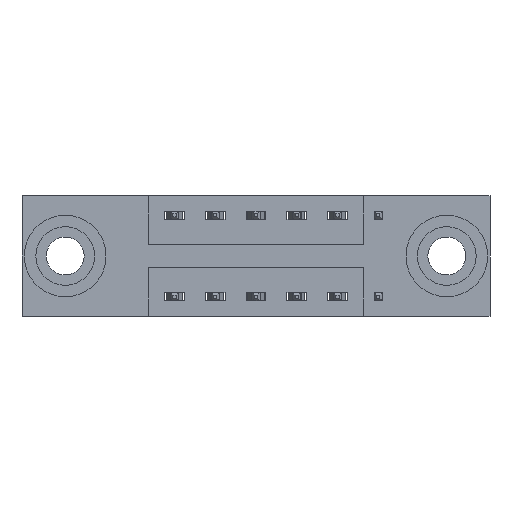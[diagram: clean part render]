
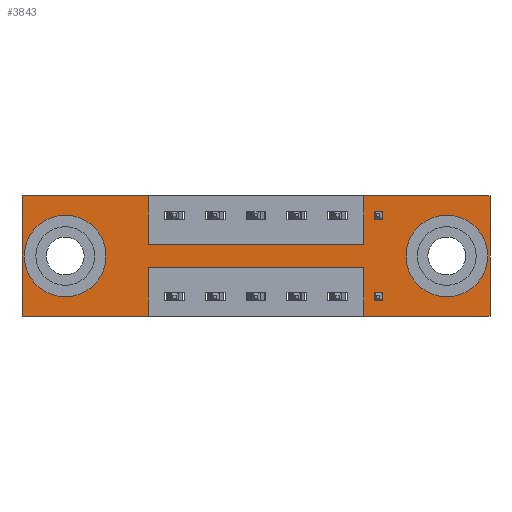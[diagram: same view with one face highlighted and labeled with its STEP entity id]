
A CAD part, front view. The second image highlights one B-rep face of the part: STEP entity #3843.
In plain terms, the highlighted planar face has unit normal (0, -1, 0).
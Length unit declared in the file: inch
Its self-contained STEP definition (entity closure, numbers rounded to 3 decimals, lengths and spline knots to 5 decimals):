
#69 = ORIENTED_EDGE ( 'NONE', *, *, #7215, .F. ) ;
#124 = DIRECTION ( 'NONE',  ( 0., 1., 0. ) ) ;
#180 = EDGE_CURVE ( 'NONE', #1295, #4848, #5429, .T. ) ;
#221 = CARTESIAN_POINT ( 'NONE',  ( 0., 0., -0.37 ) ) ;
#289 = EDGE_LOOP ( 'NONE', ( #3322, #6842, #1439, #1533, #9159, #69, #3144, #7101, #3628, #953, #3775, #3392 ) ) ;
#499 = VERTEX_POINT ( 'NONE', #5935 ) ;
#575 = DIRECTION ( 'NONE',  ( 0., 0., 1. ) ) ;
#671 = LINE ( 'NONE', #8808, #6575 ) ;
#814 = CARTESIAN_POINT ( 'NONE',  ( 0., 0., 0. ) ) ;
#820 = CARTESIAN_POINT ( 'NONE',  ( 1.0475, 0., -0.15 ) ) ;
#825 = EDGE_CURVE ( 'NONE', #3802, #5797, #4460, .T. ) ;
#881 = LINE ( 'NONE', #5229, #1136 ) ;
#882 = EDGE_CURVE ( 'NONE', #4845, #5880, #881, .T. ) ;
#922 = DIRECTION ( 'NONE',  ( 0., 0., 1. ) ) ;
#953 = ORIENTED_EDGE ( 'NONE', *, *, #7988, .F. ) ;
#956 = DIRECTION ( 'NONE',  ( -1., 0., 0. ) ) ;
#1047 = ORIENTED_EDGE ( 'NONE', *, *, #5486, .T. ) ;
#1136 = VECTOR ( 'NONE', #1576, 39.37008 ) ;
#1208 = CARTESIAN_POINT ( 'NONE',  ( 1.435, 0., -0.37 ) ) ;
#1213 = VERTEX_POINT ( 'NONE', #4296 ) ;
#1257 = EDGE_LOOP ( 'NONE', ( #1047, #8775 ) ) ;
#1295 = VERTEX_POINT ( 'NONE', #7350 ) ;
#1338 = DIRECTION ( 'NONE',  ( 0., 0., 1. ) ) ;
#1348 = DIRECTION ( 'NONE',  ( 0., 1., 0. ) ) ;
#1439 = ORIENTED_EDGE ( 'NONE', *, *, #825, .F. ) ;
#1474 = VERTEX_POINT ( 'NONE', #1208 ) ;
#1533 = ORIENTED_EDGE ( 'NONE', *, *, #3682, .F. ) ;
#1576 = DIRECTION ( 'NONE',  ( 1., 0., 0. ) ) ;
#1707 = VERTEX_POINT ( 'NONE', #9294 ) ;
#1776 = ORIENTED_EDGE ( 'NONE', *, *, #180, .T. ) ;
#1983 = EDGE_CURVE ( 'NONE', #2358, #1213, #5706, .T. ) ;
#2044 = CARTESIAN_POINT ( 'NONE',  ( 0., 0., -0.37 ) ) ;
#2072 = DIRECTION ( 'NONE',  ( 0., 0., -1. ) ) ;
#2266 = LINE ( 'NONE', #3748, #4459 ) ;
#2354 = CARTESIAN_POINT ( 'NONE',  ( 1.0475, 0., -0.37 ) ) ;
#2358 = VERTEX_POINT ( 'NONE', #4408 ) ;
#2485 = CIRCLE ( 'NONE', #9288, 0.078 ) ;
#2624 = VERTEX_POINT ( 'NONE', #6825 ) ;
#2844 = CARTESIAN_POINT ( 'NONE',  ( 0.1325, 0., -0.185 ) ) ;
#2926 = DIRECTION ( 'NONE',  ( 0., 0., -1. ) ) ;
#3001 = VECTOR ( 'NONE', #7055, 39.37008 ) ;
#3065 = DIRECTION ( 'NONE',  ( 0., 0., -1. ) ) ;
#3144 = ORIENTED_EDGE ( 'NONE', *, *, #5821, .F. ) ;
#3250 = EDGE_CURVE ( 'NONE', #7354, #1707, #6542, .T. ) ;
#3322 = ORIENTED_EDGE ( 'NONE', *, *, #3552, .F. ) ;
#3346 = FACE_OUTER_BOUND ( 'NONE', #289, .T. ) ;
#3392 = ORIENTED_EDGE ( 'NONE', *, *, #1983, .F. ) ;
#3408 = CARTESIAN_POINT ( 'NONE',  ( 0., 0., 0. ) ) ;
#3552 = EDGE_CURVE ( 'NONE', #7711, #2358, #2266, .T. ) ;
#3562 = CARTESIAN_POINT ( 'NONE',  ( 1.0475, 0., -0.22 ) ) ;
#3628 = ORIENTED_EDGE ( 'NONE', *, *, #4760, .F. ) ;
#3682 = EDGE_CURVE ( 'NONE', #1474, #3802, #3893, .T. ) ;
#3699 = EDGE_LOOP ( 'NONE', ( #8478, #1776 ) ) ;
#3748 = CARTESIAN_POINT ( 'NONE',  ( 0.3875, 0., -0.37 ) ) ;
#3775 = ORIENTED_EDGE ( 'NONE', *, *, #7913, .F. ) ;
#3802 = VERTEX_POINT ( 'NONE', #6943 ) ;
#3821 = CARTESIAN_POINT ( 'NONE',  ( 1.435, 0., 0. ) ) ;
#3843 = ADVANCED_FACE ( 'NONE', ( #8562, #9128, #3346 ), #6281, .T. ) ;
#3875 = CIRCLE ( 'NONE', #5547, 0.078 ) ;
#3893 = LINE ( 'NONE', #221, #5077 ) ;
#3953 = CARTESIAN_POINT ( 'NONE',  ( 1.3025, 0., -0.107 ) ) ;
#3959 = VECTOR ( 'NONE', #5259, 39.37008 ) ;
#4190 = DIRECTION ( 'NONE',  ( 0., 1., 0. ) ) ;
#4296 = CARTESIAN_POINT ( 'NONE',  ( 0., 0., -0.37 ) ) ;
#4347 = VECTOR ( 'NONE', #7044, 39.37008 ) ;
#4399 = CARTESIAN_POINT ( 'NONE',  ( 1.3025, 0., -0.185 ) ) ;
#4408 = CARTESIAN_POINT ( 'NONE',  ( 0.3875, 0., -0.37 ) ) ;
#4459 = VECTOR ( 'NONE', #2926, 39.37008 ) ;
#4460 = LINE ( 'NONE', #2354, #5435 ) ;
#4559 = CARTESIAN_POINT ( 'NONE',  ( 1.3025, 0., -0.185 ) ) ;
#4616 = LINE ( 'NONE', #7475, #6516 ) ;
#4716 = CARTESIAN_POINT ( 'NONE',  ( 0.3875, 0., -0.15 ) ) ;
#4757 = AXIS2_PLACEMENT_3D ( 'NONE', #2844, #4190, #1338 ) ;
#4760 = EDGE_CURVE ( 'NONE', #6452, #4845, #671, .T. ) ;
#4767 = LINE ( 'NONE', #7628, #9231 ) ;
#4845 = VERTEX_POINT ( 'NONE', #4716 ) ;
#4848 = VERTEX_POINT ( 'NONE', #3953 ) ;
#5061 = DIRECTION ( 'NONE',  ( 0., 0., -1. ) ) ;
#5065 = EDGE_CURVE ( 'NONE', #4848, #1295, #2485, .T. ) ;
#5077 = VECTOR ( 'NONE', #7505, 39.37008 ) ;
#5100 = DIRECTION ( 'NONE',  ( 0., 0., -1. ) ) ;
#5218 = CARTESIAN_POINT ( 'NONE',  ( 1.0475, 0., 0. ) ) ;
#5229 = CARTESIAN_POINT ( 'NONE',  ( 0.3875, 0., -0.15 ) ) ;
#5258 = VECTOR ( 'NONE', #922, 39.37008 ) ;
#5259 = DIRECTION ( 'NONE',  ( 0., 0., 1. ) ) ;
#5343 = LINE ( 'NONE', #814, #3959 ) ;
#5429 = CIRCLE ( 'NONE', #7054, 0.078 ) ;
#5435 = VECTOR ( 'NONE', #8832, 39.37008 ) ;
#5486 = EDGE_CURVE ( 'NONE', #1707, #7354, #3875, .T. ) ;
#5547 = AXIS2_PLACEMENT_3D ( 'NONE', #5757, #1348, #575 ) ;
#5687 = DIRECTION ( 'NONE',  ( 0., -1., 0. ) ) ;
#5706 = LINE ( 'NONE', #2044, #3001 ) ;
#5757 = CARTESIAN_POINT ( 'NONE',  ( 0.1325, 0., -0.185 ) ) ;
#5797 = VERTEX_POINT ( 'NONE', #3562 ) ;
#5821 = EDGE_CURVE ( 'NONE', #5880, #499, #8816, .T. ) ;
#5880 = VERTEX_POINT ( 'NONE', #820 ) ;
#5935 = CARTESIAN_POINT ( 'NONE',  ( 1.0475, 0., 0. ) ) ;
#6129 = EDGE_CURVE ( 'NONE', #2624, #1474, #8670, .T. ) ;
#6281 = PLANE ( 'NONE',  #7017 ) ;
#6364 = CARTESIAN_POINT ( 'NONE',  ( 0., 0., -0.37 ) ) ;
#6396 = CARTESIAN_POINT ( 'NONE',  ( 0.3875, 0., -0.22 ) ) ;
#6452 = VERTEX_POINT ( 'NONE', #6631 ) ;
#6516 = VECTOR ( 'NONE', #956, 39.37008 ) ;
#6542 = CIRCLE ( 'NONE', #4757, 0.078 ) ;
#6566 = CARTESIAN_POINT ( 'NONE',  ( 0.1325, 0., -0.263 ) ) ;
#6575 = VECTOR ( 'NONE', #5061, 39.37008 ) ;
#6631 = CARTESIAN_POINT ( 'NONE',  ( 0.3875, 0., 0. ) ) ;
#6825 = CARTESIAN_POINT ( 'NONE',  ( 1.435, 0., 0. ) ) ;
#6842 = ORIENTED_EDGE ( 'NONE', *, *, #8152, .F. ) ;
#6916 = DIRECTION ( 'NONE',  ( 1., 0., 0. ) ) ;
#6943 = CARTESIAN_POINT ( 'NONE',  ( 1.0475, 0., -0.37 ) ) ;
#7017 = AXIS2_PLACEMENT_3D ( 'NONE', #6364, #5687, #2072 ) ;
#7044 = DIRECTION ( 'NONE',  ( 1., 0., 0. ) ) ;
#7054 = AXIS2_PLACEMENT_3D ( 'NONE', #4399, #7939, #8733 ) ;
#7055 = DIRECTION ( 'NONE',  ( -1., 0., 0. ) ) ;
#7101 = ORIENTED_EDGE ( 'NONE', *, *, #882, .F. ) ;
#7215 = EDGE_CURVE ( 'NONE', #499, #2624, #7755, .T. ) ;
#7350 = CARTESIAN_POINT ( 'NONE',  ( 1.3025, 0., -0.263 ) ) ;
#7354 = VERTEX_POINT ( 'NONE', #6566 ) ;
#7475 = CARTESIAN_POINT ( 'NONE',  ( 0.3875, 0., -0.22 ) ) ;
#7505 = DIRECTION ( 'NONE',  ( -1., 0., 0. ) ) ;
#7578 = CARTESIAN_POINT ( 'NONE',  ( 0., 0., 0. ) ) ;
#7628 = CARTESIAN_POINT ( 'NONE',  ( 0., 0., 0. ) ) ;
#7711 = VERTEX_POINT ( 'NONE', #6396 ) ;
#7755 = LINE ( 'NONE', #3408, #4347 ) ;
#7913 = EDGE_CURVE ( 'NONE', #1213, #7975, #5343, .T. ) ;
#7939 = DIRECTION ( 'NONE',  ( 0., 1., 0. ) ) ;
#7975 = VERTEX_POINT ( 'NONE', #7578 ) ;
#7988 = EDGE_CURVE ( 'NONE', #7975, #6452, #4767, .T. ) ;
#8106 = VECTOR ( 'NONE', #5100, 39.37008 ) ;
#8152 = EDGE_CURVE ( 'NONE', #5797, #7711, #4616, .T. ) ;
#8478 = ORIENTED_EDGE ( 'NONE', *, *, #5065, .T. ) ;
#8562 = FACE_BOUND ( 'NONE', #3699, .T. ) ;
#8670 = LINE ( 'NONE', #3821, #8106 ) ;
#8733 = DIRECTION ( 'NONE',  ( 0., 0., -1. ) ) ;
#8775 = ORIENTED_EDGE ( 'NONE', *, *, #3250, .T. ) ;
#8808 = CARTESIAN_POINT ( 'NONE',  ( 0.3875, 0., 0. ) ) ;
#8816 = LINE ( 'NONE', #5218, #5258 ) ;
#8832 = DIRECTION ( 'NONE',  ( 0., 0., 1. ) ) ;
#9128 = FACE_BOUND ( 'NONE', #1257, .T. ) ;
#9159 = ORIENTED_EDGE ( 'NONE', *, *, #6129, .F. ) ;
#9231 = VECTOR ( 'NONE', #6916, 39.37008 ) ;
#9288 = AXIS2_PLACEMENT_3D ( 'NONE', #4559, #124, #3065 ) ;
#9294 = CARTESIAN_POINT ( 'NONE',  ( 0.1325, 0., -0.107 ) ) ;
